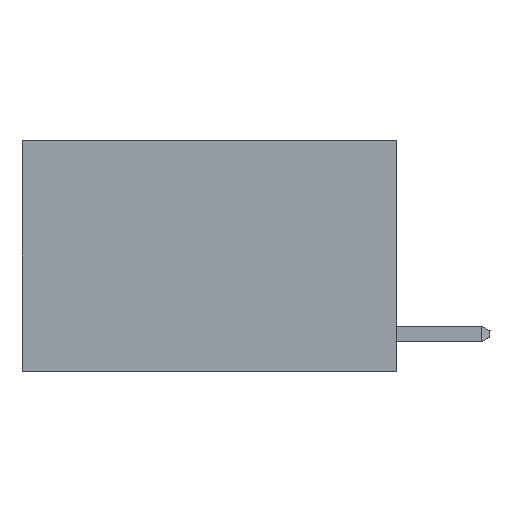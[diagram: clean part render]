
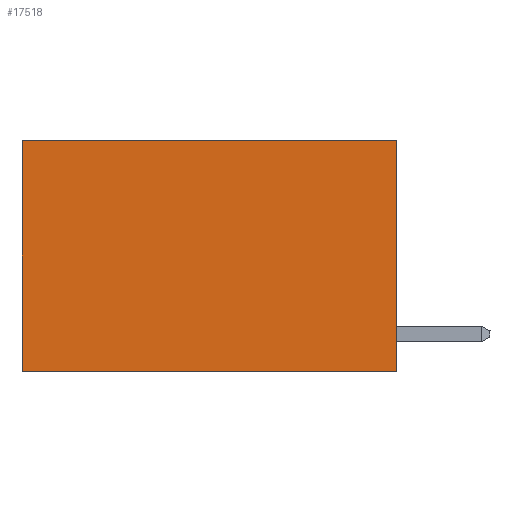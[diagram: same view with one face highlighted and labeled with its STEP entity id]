
A CAD part, left-side view. The second image highlights one B-rep face of the part: STEP entity #17518.
In plain terms, the highlighted planar face has unit normal (-1, 0, 0).
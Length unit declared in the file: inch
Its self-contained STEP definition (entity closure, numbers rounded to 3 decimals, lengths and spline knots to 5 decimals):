
#1325 = CARTESIAN_POINT ( 'NONE',  ( 0.2625, 0., 0. ) ) ;
#2106 = DIRECTION ( 'NONE',  ( 0., 1., 0. ) ) ;
#2293 = VERTEX_POINT ( 'NONE', #2550 ) ;
#2550 = CARTESIAN_POINT ( 'NONE',  ( 0.2625, 0.6, 0. ) ) ;
#2560 = EDGE_CURVE ( 'NONE', #17273, #2293, #13082, .T. ) ;
#2627 = PLANE ( 'NONE',  #7078 ) ;
#3015 = CARTESIAN_POINT ( 'NONE',  ( 0.2625, 0., 0. ) ) ;
#3366 = VECTOR ( 'NONE', #5447, 39.37008 ) ;
#3496 = VECTOR ( 'NONE', #2106, 39.37008 ) ;
#3607 = DIRECTION ( 'NONE',  ( 0., 0., -1. ) ) ;
#3834 = LINE ( 'NONE', #12322, #17370 ) ;
#5191 = ORIENTED_EDGE ( 'NONE', *, *, #17994, .T. ) ;
#5447 = DIRECTION ( 'NONE',  ( 0., 0., -1. ) ) ;
#5541 = EDGE_LOOP ( 'NONE', ( #5191, #12056, #7070, #10087 ) ) ;
#6154 = CARTESIAN_POINT ( 'NONE',  ( 0.2625, 0., 0. ) ) ;
#6755 = DIRECTION ( 'NONE',  ( 0., 1., 0. ) ) ;
#7070 = ORIENTED_EDGE ( 'NONE', *, *, #7417, .F. ) ;
#7077 = DIRECTION ( 'NONE',  ( 0., 0., -1. ) ) ;
#7078 = AXIS2_PLACEMENT_3D ( 'NONE', #7935, #17815, #7077 ) ;
#7417 = EDGE_CURVE ( 'NONE', #17273, #8418, #10817, .T. ) ;
#7935 = CARTESIAN_POINT ( 'NONE',  ( 0.2625, 0., 0. ) ) ;
#8418 = VERTEX_POINT ( 'NONE', #8532 ) ;
#8532 = CARTESIAN_POINT ( 'NONE',  ( 0.2625, 0., -0.37 ) ) ;
#8810 = CARTESIAN_POINT ( 'NONE',  ( 0.2625, 0.6, -0.37 ) ) ;
#9385 = CARTESIAN_POINT ( 'NONE',  ( 0.2625, 0.6, 0. ) ) ;
#10087 = ORIENTED_EDGE ( 'NONE', *, *, #2560, .T. ) ;
#10382 = FACE_OUTER_BOUND ( 'NONE', #5541, .T. ) ;
#10576 = LINE ( 'NONE', #9385, #16893 ) ;
#10817 = LINE ( 'NONE', #1325, #3366 ) ;
#12056 = ORIENTED_EDGE ( 'NONE', *, *, #17168, .F. ) ;
#12086 = VERTEX_POINT ( 'NONE', #8810 ) ;
#12322 = CARTESIAN_POINT ( 'NONE',  ( 0.2625, 0., -0.37 ) ) ;
#13082 = LINE ( 'NONE', #6154, #3496 ) ;
#16893 = VECTOR ( 'NONE', #3607, 39.37008 ) ;
#17168 = EDGE_CURVE ( 'NONE', #8418, #12086, #3834, .T. ) ;
#17273 = VERTEX_POINT ( 'NONE', #3015 ) ;
#17370 = VECTOR ( 'NONE', #6755, 39.37008 ) ;
#17518 = ADVANCED_FACE ( 'NONE', ( #10382 ), #2627, .F. ) ;
#17815 = DIRECTION ( 'NONE',  ( 1., 0., 0. ) ) ;
#17994 = EDGE_CURVE ( 'NONE', #2293, #12086, #10576, .T. ) ;
